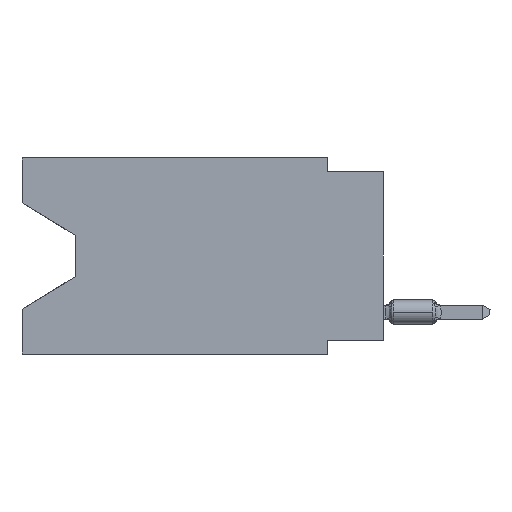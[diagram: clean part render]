
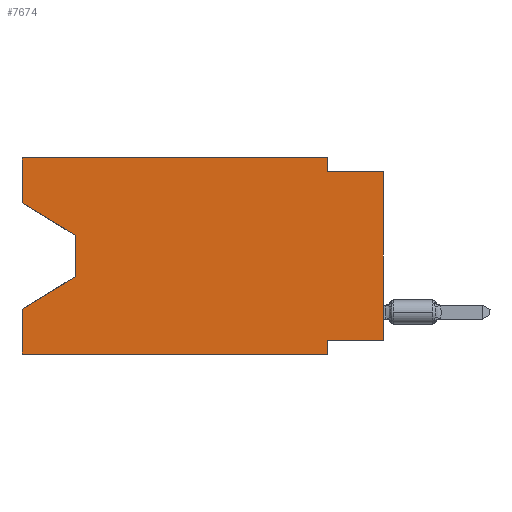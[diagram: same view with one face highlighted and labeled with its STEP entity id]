
A CAD part, left-side view. The second image highlights one B-rep face of the part: STEP entity #7674.
In plain terms, the highlighted planar face has unit normal (-1, 0, 0).
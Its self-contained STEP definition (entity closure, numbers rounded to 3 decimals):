
#737 = CARTESIAN_POINT ( 'NONE',  ( 0., 16.383, 0. ) ) ;
#1089 = PLANE ( 'NONE',  #53225 ) ;
#1724 = CARTESIAN_POINT ( 'NONE',  ( 0., 2.54, -8.89 ) ) ;
#2356 = EDGE_CURVE ( 'NONE', #7235, #4073, #46808, .T. ) ;
#3379 = CARTESIAN_POINT ( 'NONE',  ( 0., 2.54, -8.89 ) ) ;
#4073 = VERTEX_POINT ( 'NONE', #57615 ) ;
#5051 = VERTEX_POINT ( 'NONE', #48364 ) ;
#5163 = LINE ( 'NONE', #9401, #26418 ) ;
#5579 = EDGE_CURVE ( 'NONE', #5051, #52452, #52008, .T. ) ;
#6911 = VECTOR ( 'NONE', #59154, 1000. ) ;
#7122 = VERTEX_POINT ( 'NONE', #23165 ) ;
#7235 = VERTEX_POINT ( 'NONE', #53625 ) ;
#7674 = ADVANCED_FACE ( 'NONE', ( #56215 ), #1089, .F. ) ;
#8900 = VECTOR ( 'NONE', #28581, 1000. ) ;
#8991 = CARTESIAN_POINT ( 'NONE',  ( 0., 16.383, -2.038 ) ) ;
#8997 = VECTOR ( 'NONE', #51911, 1000. ) ;
#9347 = EDGE_CURVE ( 'NONE', #9520, #7122, #51312, .T. ) ;
#9401 = CARTESIAN_POINT ( 'NONE',  ( 0., 16.383, -8.89 ) ) ;
#9520 = VERTEX_POINT ( 'NONE', #8991 ) ;
#9574 = CARTESIAN_POINT ( 'NONE',  ( 0., 16.383, 0. ) ) ;
#9779 = CARTESIAN_POINT ( 'NONE',  ( 0., 0., -8.255 ) ) ;
#9824 = DIRECTION ( 'NONE',  ( 0., 0., 1. ) ) ;
#12264 = DIRECTION ( 'NONE',  ( 0., -0.855, -0.519 ) ) ;
#13123 = CARTESIAN_POINT ( 'NONE',  ( 0., 16.383, 0. ) ) ;
#13398 = ORIENTED_EDGE ( 'NONE', *, *, #48263, .T. ) ;
#13464 = CARTESIAN_POINT ( 'NONE',  ( 0., 16.383, -2.038 ) ) ;
#13760 = CARTESIAN_POINT ( 'NONE',  ( 0., 13.97, -3.505 ) ) ;
#14140 = VERTEX_POINT ( 'NONE', #20458 ) ;
#14733 = DIRECTION ( 'NONE',  ( 1., 0., 0. ) ) ;
#14856 = DIRECTION ( 'NONE',  ( 0., -1., 0. ) ) ;
#15416 = VECTOR ( 'NONE', #37480, 1000. ) ;
#16824 = LINE ( 'NONE', #13464, #43704 ) ;
#17068 = LINE ( 'NONE', #13123, #6911 ) ;
#17516 = DIRECTION ( 'NONE',  ( 0., 0., -1. ) ) ;
#18089 = EDGE_LOOP ( 'NONE', ( #13398, #44227, #21748, #34182, #47916, #39819, #44566, #35216, #35864, #43855, #34702, #50077 ) ) ;
#18376 = DIRECTION ( 'NONE',  ( 0., 0., -1. ) ) ;
#18900 = LINE ( 'NONE', #19497, #47052 ) ;
#19497 = CARTESIAN_POINT ( 'NONE',  ( 0., 16.383, 0. ) ) ;
#20020 = VERTEX_POINT ( 'NONE', #28652 ) ;
#20458 = CARTESIAN_POINT ( 'NONE',  ( 0., 2.54, 0. ) ) ;
#20530 = VECTOR ( 'NONE', #17516, 1000. ) ;
#20747 = EDGE_CURVE ( 'NONE', #53677, #31078, #59438, .T. ) ;
#21147 = EDGE_CURVE ( 'NONE', #7122, #14140, #18900, .T. ) ;
#21748 = ORIENTED_EDGE ( 'NONE', *, *, #2356, .T. ) ;
#23155 = LINE ( 'NONE', #28883, #53082 ) ;
#23165 = CARTESIAN_POINT ( 'NONE',  ( 0., 16.383, 0. ) ) ;
#26011 = CARTESIAN_POINT ( 'NONE',  ( 0., 0., -0.635 ) ) ;
#26418 = VECTOR ( 'NONE', #14856, 1000. ) ;
#27960 = LINE ( 'NONE', #9779, #51394 ) ;
#28581 = DIRECTION ( 'NONE',  ( 0., 0., -1. ) ) ;
#28631 = CARTESIAN_POINT ( 'NONE',  ( 0., 13.97, -5.385 ) ) ;
#28652 = CARTESIAN_POINT ( 'NONE',  ( 0., 0., -8.255 ) ) ;
#28883 = CARTESIAN_POINT ( 'NONE',  ( 0., 0., 0. ) ) ;
#31078 = VERTEX_POINT ( 'NONE', #26011 ) ;
#31367 = VERTEX_POINT ( 'NONE', #56856 ) ;
#32918 = EDGE_CURVE ( 'NONE', #20020, #5051, #27960, .T. ) ;
#33139 = LINE ( 'NONE', #51291, #8900 ) ;
#33162 = EDGE_CURVE ( 'NONE', #31367, #4073, #17068, .T. ) ;
#34031 = EDGE_CURVE ( 'NONE', #14140, #53677, #44776, .T. ) ;
#34182 = ORIENTED_EDGE ( 'NONE', *, *, #33162, .F. ) ;
#34702 = ORIENTED_EDGE ( 'NONE', *, *, #21147, .F. ) ;
#35216 = ORIENTED_EDGE ( 'NONE', *, *, #51779, .T. ) ;
#35528 = VECTOR ( 'NONE', #41256, 1000. ) ;
#35864 = ORIENTED_EDGE ( 'NONE', *, *, #20747, .F. ) ;
#37480 = DIRECTION ( 'NONE',  ( 0., 0., -1. ) ) ;
#39819 = ORIENTED_EDGE ( 'NONE', *, *, #5579, .F. ) ;
#40348 = CARTESIAN_POINT ( 'NONE',  ( 0., 0., -0.635 ) ) ;
#40949 = CARTESIAN_POINT ( 'NONE',  ( 0., 2.54, -0.635 ) ) ;
#41256 = DIRECTION ( 'NONE',  ( 0., -1., 0. ) ) ;
#43704 = VECTOR ( 'NONE', #12264, 1000. ) ;
#43855 = ORIENTED_EDGE ( 'NONE', *, *, #34031, .F. ) ;
#44227 = ORIENTED_EDGE ( 'NONE', *, *, #50506, .T. ) ;
#44305 = EDGE_CURVE ( 'NONE', #31367, #52452, #5163, .T. ) ;
#44566 = ORIENTED_EDGE ( 'NONE', *, *, #32918, .F. ) ;
#44776 = LINE ( 'NONE', #57823, #20530 ) ;
#46425 = DIRECTION ( 'NONE',  ( 0., 1., 0. ) ) ;
#46808 = LINE ( 'NONE', #28631, #53847 ) ;
#47052 = VECTOR ( 'NONE', #47333, 1000. ) ;
#47209 = VERTEX_POINT ( 'NONE', #13760 ) ;
#47333 = DIRECTION ( 'NONE',  ( 0., -1., 0. ) ) ;
#47916 = ORIENTED_EDGE ( 'NONE', *, *, #44305, .T. ) ;
#48263 = EDGE_CURVE ( 'NONE', #9520, #47209, #16824, .T. ) ;
#48364 = CARTESIAN_POINT ( 'NONE',  ( 0., 2.54, -8.255 ) ) ;
#50077 = ORIENTED_EDGE ( 'NONE', *, *, #9347, .F. ) ;
#50506 = EDGE_CURVE ( 'NONE', #47209, #7235, #33139, .T. ) ;
#51044 = DIRECTION ( 'NONE',  ( 0., 0.855, -0.519 ) ) ;
#51291 = CARTESIAN_POINT ( 'NONE',  ( 0., 13.97, -3.505 ) ) ;
#51312 = LINE ( 'NONE', #737, #8997 ) ;
#51394 = VECTOR ( 'NONE', #46425, 1000. ) ;
#51779 = EDGE_CURVE ( 'NONE', #20020, #31078, #23155, .T. ) ;
#51911 = DIRECTION ( 'NONE',  ( 0., 0., 1. ) ) ;
#52008 = LINE ( 'NONE', #1724, #15416 ) ;
#52452 = VERTEX_POINT ( 'NONE', #3379 ) ;
#53082 = VECTOR ( 'NONE', #9824, 1000. ) ;
#53225 = AXIS2_PLACEMENT_3D ( 'NONE', #9574, #14733, #18376 ) ;
#53625 = CARTESIAN_POINT ( 'NONE',  ( 0., 13.97, -5.385 ) ) ;
#53677 = VERTEX_POINT ( 'NONE', #40949 ) ;
#53847 = VECTOR ( 'NONE', #51044, 1000. ) ;
#56215 = FACE_OUTER_BOUND ( 'NONE', #18089, .T. ) ;
#56856 = CARTESIAN_POINT ( 'NONE',  ( 0., 16.383, -8.89 ) ) ;
#57615 = CARTESIAN_POINT ( 'NONE',  ( 0., 16.383, -6.852 ) ) ;
#57823 = CARTESIAN_POINT ( 'NONE',  ( 0., 2.54, 0. ) ) ;
#59154 = DIRECTION ( 'NONE',  ( 0., 0., 1. ) ) ;
#59438 = LINE ( 'NONE', #40348, #35528 ) ;
